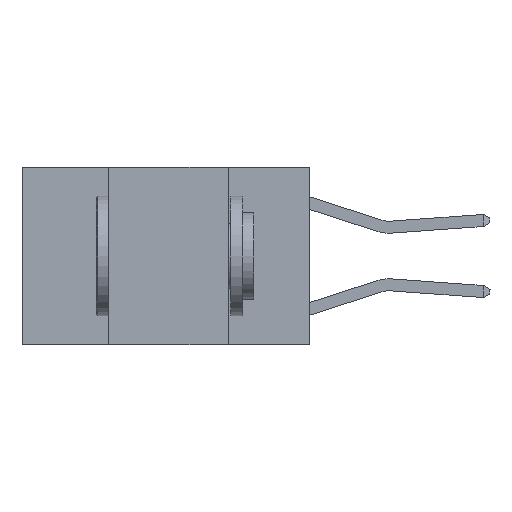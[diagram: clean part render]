
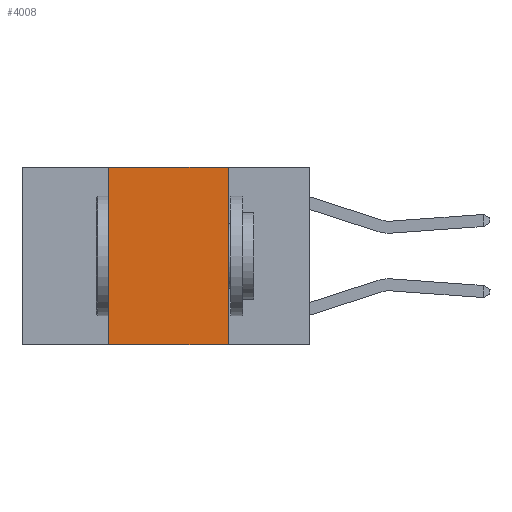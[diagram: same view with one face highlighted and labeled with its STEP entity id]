
A CAD part, left-side view. The second image highlights one B-rep face of the part: STEP entity #4008.
In plain terms, the highlighted planar face has unit normal (-1, 0, 0).
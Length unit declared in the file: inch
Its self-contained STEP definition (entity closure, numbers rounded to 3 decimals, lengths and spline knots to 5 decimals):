
#274 = LINE ( 'NONE', #4723, #9021 ) ;
#490 = DIRECTION ( 'NONE',  ( 0., 0., -1. ) ) ;
#548 = LINE ( 'NONE', #5933, #7548 ) ;
#757 = CARTESIAN_POINT ( 'NONE',  ( 0., 0.17, 0. ) ) ;
#1409 = ORIENTED_EDGE ( 'NONE', *, *, #8376, .F. ) ;
#1599 = DIRECTION ( 'NONE',  ( 0., -1., 0. ) ) ;
#1692 = ORIENTED_EDGE ( 'NONE', *, *, #7866, .T. ) ;
#1755 = EDGE_CURVE ( 'NONE', #7101, #2647, #9730, .T. ) ;
#2058 = PLANE ( 'NONE',  #2269 ) ;
#2084 = VERTEX_POINT ( 'NONE', #9693 ) ;
#2269 = AXIS2_PLACEMENT_3D ( 'NONE', #7151, #8173, #2940 ) ;
#2309 = EDGE_LOOP ( 'NONE', ( #8141, #1409, #6095, #1692 ) ) ;
#2531 = VERTEX_POINT ( 'NONE', #10731 ) ;
#2647 = VERTEX_POINT ( 'NONE', #9301 ) ;
#2838 = VECTOR ( 'NONE', #490, 39.37008 ) ;
#2940 = DIRECTION ( 'NONE',  ( 0., 0., -1. ) ) ;
#3905 = CARTESIAN_POINT ( 'NONE',  ( 0., 0.17, 0. ) ) ;
#4008 = ADVANCED_FACE ( 'NONE', ( #6070 ), #2058, .F. ) ;
#4723 = CARTESIAN_POINT ( 'NONE',  ( 0., 0.6, -0.37 ) ) ;
#5933 = CARTESIAN_POINT ( 'NONE',  ( 0., 0.6, 0. ) ) ;
#6070 = FACE_OUTER_BOUND ( 'NONE', #2309, .T. ) ;
#6095 = ORIENTED_EDGE ( 'NONE', *, *, #7947, .F. ) ;
#6191 = VECTOR ( 'NONE', #10811, 39.37008 ) ;
#7101 = VERTEX_POINT ( 'NONE', #3905 ) ;
#7151 = CARTESIAN_POINT ( 'NONE',  ( 0., 0.6, 0. ) ) ;
#7548 = VECTOR ( 'NONE', #1599, 39.37008 ) ;
#7866 = EDGE_CURVE ( 'NONE', #2084, #2647, #274, .T. ) ;
#7947 = EDGE_CURVE ( 'NONE', #2084, #2531, #8499, .T. ) ;
#8141 = ORIENTED_EDGE ( 'NONE', *, *, #1755, .F. ) ;
#8173 = DIRECTION ( 'NONE',  ( 1., 0., 0. ) ) ;
#8318 = CARTESIAN_POINT ( 'NONE',  ( 0., 0.42, 0. ) ) ;
#8376 = EDGE_CURVE ( 'NONE', #2531, #7101, #548, .T. ) ;
#8499 = LINE ( 'NONE', #8318, #6191 ) ;
#9021 = VECTOR ( 'NONE', #10704, 39.37008 ) ;
#9301 = CARTESIAN_POINT ( 'NONE',  ( 0., 0.17, -0.37 ) ) ;
#9693 = CARTESIAN_POINT ( 'NONE',  ( 0., 0.42, -0.37 ) ) ;
#9730 = LINE ( 'NONE', #757, #2838 ) ;
#10704 = DIRECTION ( 'NONE',  ( 0., -1., 0. ) ) ;
#10731 = CARTESIAN_POINT ( 'NONE',  ( 0., 0.42, 0. ) ) ;
#10811 = DIRECTION ( 'NONE',  ( 0., 0., 1. ) ) ;
